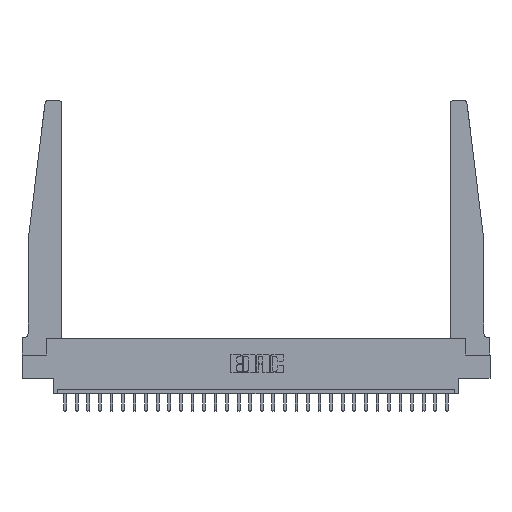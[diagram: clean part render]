
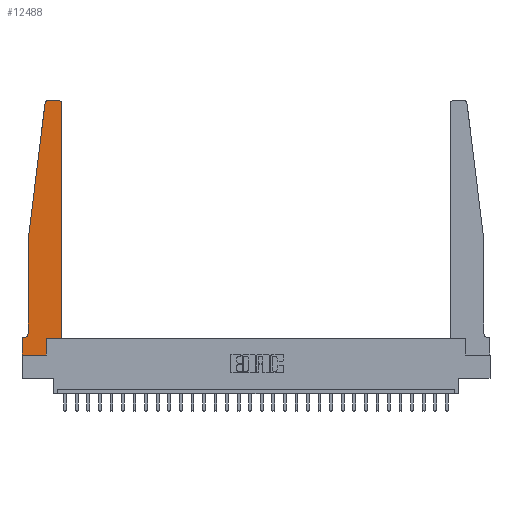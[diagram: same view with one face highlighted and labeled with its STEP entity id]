
A CAD part, top view. The second image highlights one B-rep face of the part: STEP entity #12488.
In plain terms, the highlighted planar face has unit normal (0, 0, 1).
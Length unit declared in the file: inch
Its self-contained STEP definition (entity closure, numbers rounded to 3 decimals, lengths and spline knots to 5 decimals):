
#48 = CARTESIAN_POINT ( 'NONE',  ( 0.2605, 0.18, 0.37 ) ) ;
#814 = CARTESIAN_POINT ( 'NONE',  ( 0.2605, 0.18, 0.37 ) ) ;
#1114 = CARTESIAN_POINT ( 'NONE',  ( 0.2605, 0., 0.37 ) ) ;
#1707 = CARTESIAN_POINT ( 'NONE',  ( 0., 0., 0.37 ) ) ;
#2240 = EDGE_CURVE ( 'NONE', #10950, #20222, #8437, .T. ) ;
#2312 = VERTEX_POINT ( 'NONE', #4738 ) ;
#2928 = DIRECTION ( 'NONE',  ( 1., 0., 0. ) ) ;
#3224 = DIRECTION ( 'NONE',  ( -1., 0., 0. ) ) ;
#3619 = CARTESIAN_POINT ( 'NONE',  ( 0.395, 2.72, 0.37 ) ) ;
#4053 = EDGE_CURVE ( 'NONE', #20222, #20457, #11137, .T. ) ;
#4289 = CARTESIAN_POINT ( 'NONE',  ( 0.065, 1.25, 0.37 ) ) ;
#4738 = CARTESIAN_POINT ( 'NONE',  ( 0.425, 0.18, 0.37 ) ) ;
#5107 = VECTOR ( 'NONE', #15130, 39.37008 ) ;
#5301 = DIRECTION ( 'NONE',  ( 0., 0., 1. ) ) ;
#5437 = CARTESIAN_POINT ( 'NONE',  ( 0., 0.1875, 0.37 ) ) ;
#5481 = ORIENTED_EDGE ( 'NONE', *, *, #21573, .T. ) ;
#5943 = CARTESIAN_POINT ( 'NONE',  ( 0.065, 1.25, 0.37 ) ) ;
#6054 = CARTESIAN_POINT ( 'NONE',  ( 0.395, 2.75, 0.37 ) ) ;
#6412 = CARTESIAN_POINT ( 'NONE',  ( 0.065, 1.25, 0.37 ) ) ;
#6577 = ORIENTED_EDGE ( 'NONE', *, *, #7552, .T. ) ;
#6951 = ORIENTED_EDGE ( 'NONE', *, *, #4053, .T. ) ;
#7552 = EDGE_CURVE ( 'NONE', #17940, #15001, #9819, .T. ) ;
#8020 = ORIENTED_EDGE ( 'NONE', *, *, #22501, .T. ) ;
#8170 = CIRCLE ( 'NONE', #12227, 0.03 ) ;
#8437 = CIRCLE ( 'NONE', #24037, 0.03 ) ;
#8457 = LINE ( 'NONE', #48, #10001 ) ;
#8805 = EDGE_LOOP ( 'NONE', ( #6951, #26874, #20561, #24231, #5481, #18488, #6577, #8020, #14381, #27287, #17513, #9590 ) ) ;
#8854 = CARTESIAN_POINT ( 'NONE',  ( 0.065, 0.2375, 0.37 ) ) ;
#9249 = LINE ( 'NONE', #26146, #17238 ) ;
#9395 = VERTEX_POINT ( 'NONE', #814 ) ;
#9590 = ORIENTED_EDGE ( 'NONE', *, *, #2240, .T. ) ;
#9819 = LINE ( 'NONE', #18321, #11121 ) ;
#10001 = VECTOR ( 'NONE', #16951, 39.37008 ) ;
#10047 = DIRECTION ( 'NONE',  ( 0., 0., 1. ) ) ;
#10100 = EDGE_CURVE ( 'NONE', #24958, #9395, #8457, .T. ) ;
#10232 = EDGE_CURVE ( 'NONE', #20457, #18099, #8170, .T. ) ;
#10532 = CARTESIAN_POINT ( 'NONE',  ( 0., 0., 0.37 ) ) ;
#10708 = DIRECTION ( 'NONE',  ( -1., 0., 0. ) ) ;
#10824 = DIRECTION ( 'NONE',  ( 0., 0., 1. ) ) ;
#10950 = VERTEX_POINT ( 'NONE', #21205 ) ;
#11121 = VECTOR ( 'NONE', #26860, 39.37008 ) ;
#11137 = LINE ( 'NONE', #21160, #18292 ) ;
#11224 = CIRCLE ( 'NONE', #18787, 0.05 ) ;
#11562 = EDGE_CURVE ( 'NONE', #2312, #10950, #26188, .T. ) ;
#12227 = AXIS2_PLACEMENT_3D ( 'NONE', #13335, #10824, #24215 ) ;
#12276 = CARTESIAN_POINT ( 'NONE',  ( 0.015, 0.2375, 0.37 ) ) ;
#12488 = ADVANCED_FACE ( 'NONE', ( #24431 ), #14064, .T. ) ;
#12550 = DIRECTION ( 'NONE',  ( 0., 0., -1. ) ) ;
#13120 = VERTEX_POINT ( 'NONE', #4289 ) ;
#13335 = CARTESIAN_POINT ( 'NONE',  ( 0.27653, 2.72, 0.37 ) ) ;
#13941 = VERTEX_POINT ( 'NONE', #19432 ) ;
#14064 = PLANE ( 'NONE',  #26125 ) ;
#14087 = EDGE_CURVE ( 'NONE', #9395, #2312, #9249, .T. ) ;
#14381 = ORIENTED_EDGE ( 'NONE', *, *, #10100, .T. ) ;
#15001 = VERTEX_POINT ( 'NONE', #1707 ) ;
#15130 = DIRECTION ( 'NONE',  ( 0., 1., 0. ) ) ;
#15626 = CARTESIAN_POINT ( 'NONE',  ( 0., 0.1875, 0.37 ) ) ;
#16583 = VECTOR ( 'NONE', #19173, 39.37008 ) ;
#16689 = LINE ( 'NONE', #5943, #20047 ) ;
#16951 = DIRECTION ( 'NONE',  ( 0., 1., 0. ) ) ;
#16994 = LINE ( 'NONE', #6412, #20438 ) ;
#17155 = VERTEX_POINT ( 'NONE', #8854 ) ;
#17238 = VECTOR ( 'NONE', #26288, 39.37008 ) ;
#17513 = ORIENTED_EDGE ( 'NONE', *, *, #11562, .T. ) ;
#17940 = VERTEX_POINT ( 'NONE', #5437 ) ;
#18099 = VERTEX_POINT ( 'NONE', #23143 ) ;
#18172 = EDGE_CURVE ( 'NONE', #13120, #17155, #16994, .T. ) ;
#18292 = VECTOR ( 'NONE', #10708, 39.37008 ) ;
#18321 = CARTESIAN_POINT ( 'NONE',  ( 0., 0., 0.37 ) ) ;
#18488 = ORIENTED_EDGE ( 'NONE', *, *, #26167, .T. ) ;
#18555 = DIRECTION ( 'NONE',  ( 1., 0., 0. ) ) ;
#18787 = AXIS2_PLACEMENT_3D ( 'NONE', #12276, #12550, #23019 ) ;
#19173 = DIRECTION ( 'NONE',  ( 1., 0., 0. ) ) ;
#19223 = DIRECTION ( 'NONE',  ( 0., -1., 0. ) ) ;
#19359 = VECTOR ( 'NONE', #3224, 39.37008 ) ;
#19432 = CARTESIAN_POINT ( 'NONE',  ( 0.015, 0.1875, 0.37 ) ) ;
#19714 = CARTESIAN_POINT ( 'NONE',  ( 0.27653, 2.75, 0.37 ) ) ;
#19950 = EDGE_CURVE ( 'NONE', #18099, #13120, #16689, .T. ) ;
#20047 = VECTOR ( 'NONE', #21145, 39.37008 ) ;
#20222 = VERTEX_POINT ( 'NONE', #6054 ) ;
#20438 = VECTOR ( 'NONE', #19223, 39.37008 ) ;
#20457 = VERTEX_POINT ( 'NONE', #19714 ) ;
#20561 = ORIENTED_EDGE ( 'NONE', *, *, #19950, .T. ) ;
#21145 = DIRECTION ( 'NONE',  ( -0.122, -0.992, 0. ) ) ;
#21160 = CARTESIAN_POINT ( 'NONE',  ( 0.25, 2.75, 0.37 ) ) ;
#21205 = CARTESIAN_POINT ( 'NONE',  ( 0.425, 2.72, 0.37 ) ) ;
#21411 = LINE ( 'NONE', #10532, #16583 ) ;
#21573 = EDGE_CURVE ( 'NONE', #17155, #13941, #11224, .T. ) ;
#22501 = EDGE_CURVE ( 'NONE', #15001, #24958, #21411, .T. ) ;
#23019 = DIRECTION ( 'NONE',  ( -1., 0., 0. ) ) ;
#23143 = CARTESIAN_POINT ( 'NONE',  ( 0.24675, 2.72367, 0.37 ) ) ;
#24037 = AXIS2_PLACEMENT_3D ( 'NONE', #3619, #10047, #18555 ) ;
#24215 = DIRECTION ( 'NONE',  ( 1., 0., 0. ) ) ;
#24231 = ORIENTED_EDGE ( 'NONE', *, *, #18172, .T. ) ;
#24431 = FACE_OUTER_BOUND ( 'NONE', #8805, .T. ) ;
#24708 = CARTESIAN_POINT ( 'NONE',  ( 0.065, 0.1875, 0.37 ) ) ;
#24958 = VERTEX_POINT ( 'NONE', #1114 ) ;
#26045 = CARTESIAN_POINT ( 'NONE',  ( 0.425, 0.18, 0.37 ) ) ;
#26125 = AXIS2_PLACEMENT_3D ( 'NONE', #15626, #5301, #2928 ) ;
#26146 = CARTESIAN_POINT ( 'NONE',  ( 0.425, 0.18, 0.37 ) ) ;
#26167 = EDGE_CURVE ( 'NONE', #13941, #17940, #26575, .T. ) ;
#26188 = LINE ( 'NONE', #26045, #5107 ) ;
#26288 = DIRECTION ( 'NONE',  ( 1., 0., 0. ) ) ;
#26575 = LINE ( 'NONE', #24708, #19359 ) ;
#26860 = DIRECTION ( 'NONE',  ( 0., -1., 0. ) ) ;
#26874 = ORIENTED_EDGE ( 'NONE', *, *, #10232, .T. ) ;
#27287 = ORIENTED_EDGE ( 'NONE', *, *, #14087, .T. ) ;
